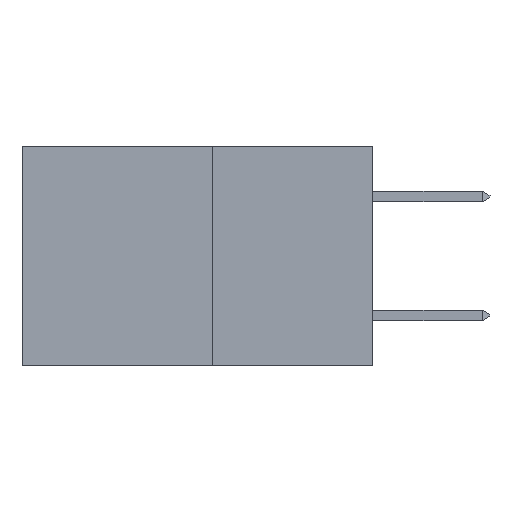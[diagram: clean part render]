
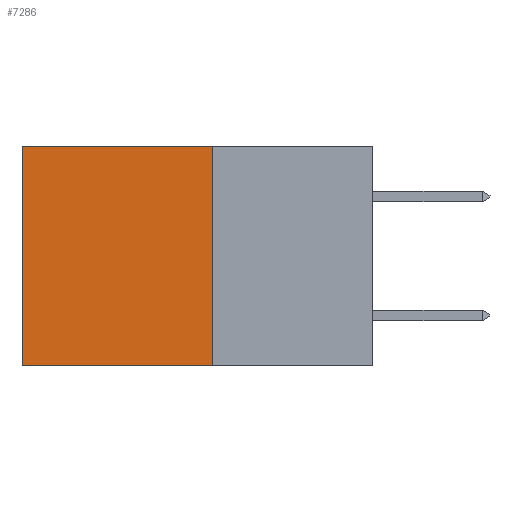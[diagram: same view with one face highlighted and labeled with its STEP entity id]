
A CAD part, left-side view. The second image highlights one B-rep face of the part: STEP entity #7286.
In plain terms, the highlighted planar face has unit normal (-1, 0, 0).
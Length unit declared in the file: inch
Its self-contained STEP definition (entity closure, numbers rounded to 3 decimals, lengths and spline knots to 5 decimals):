
#212 = LINE ( 'NONE', #3777, #11324 ) ;
#444 = CARTESIAN_POINT ( 'NONE',  ( 0.277, 0.27, -0.37 ) ) ;
#1114 = ORIENTED_EDGE ( 'NONE', *, *, #1220, .F. ) ;
#1220 = EDGE_CURVE ( 'NONE', #12785, #11777, #10015, .T. ) ;
#1423 = VERTEX_POINT ( 'NONE', #11241 ) ;
#1479 = AXIS2_PLACEMENT_3D ( 'NONE', #10381, #12316, #6412 ) ;
#1875 = FACE_OUTER_BOUND ( 'NONE', #11082, .T. ) ;
#2586 = LINE ( 'NONE', #10477, #10110 ) ;
#2786 = VERTEX_POINT ( 'NONE', #11202 ) ;
#3022 = EDGE_CURVE ( 'NONE', #2786, #12785, #11637, .T. ) ;
#3646 = CARTESIAN_POINT ( 'NONE',  ( 0.277, 0.27, -0.37 ) ) ;
#3752 = EDGE_CURVE ( 'NONE', #2786, #1423, #212, .T. ) ;
#3777 = CARTESIAN_POINT ( 'NONE',  ( 0.277, 0.27, 0. ) ) ;
#4813 = DIRECTION ( 'NONE',  ( 0., 1., 0. ) ) ;
#5529 = DIRECTION ( 'NONE',  ( 0., 0., -1. ) ) ;
#5591 = CARTESIAN_POINT ( 'NONE',  ( 0.277, 0.59, -0.37 ) ) ;
#6346 = VECTOR ( 'NONE', #10533, 39.37008 ) ;
#6412 = DIRECTION ( 'NONE',  ( 0., 0., -1. ) ) ;
#6817 = ORIENTED_EDGE ( 'NONE', *, *, #3022, .F. ) ;
#7286 = ADVANCED_FACE ( 'NONE', ( #1875 ), #9343, .F. ) ;
#9343 = PLANE ( 'NONE',  #1479 ) ;
#9415 = ORIENTED_EDGE ( 'NONE', *, *, #3752, .T. ) ;
#9535 = CARTESIAN_POINT ( 'NONE',  ( 0.277, 0.27, -0.37 ) ) ;
#9672 = VECTOR ( 'NONE', #12579, 39.37008 ) ;
#10015 = LINE ( 'NONE', #444, #9672 ) ;
#10110 = VECTOR ( 'NONE', #5529, 39.37008 ) ;
#10329 = EDGE_CURVE ( 'NONE', #1423, #11777, #2586, .T. ) ;
#10381 = CARTESIAN_POINT ( 'NONE',  ( 0.277, 0.27, -0.37 ) ) ;
#10477 = CARTESIAN_POINT ( 'NONE',  ( 0.277, 0.59, -0.37 ) ) ;
#10533 = DIRECTION ( 'NONE',  ( 0., 0., -1. ) ) ;
#11082 = EDGE_LOOP ( 'NONE', ( #11769, #1114, #6817, #9415 ) ) ;
#11202 = CARTESIAN_POINT ( 'NONE',  ( 0.277, 0.27, 0. ) ) ;
#11241 = CARTESIAN_POINT ( 'NONE',  ( 0.277, 0.59, 0. ) ) ;
#11324 = VECTOR ( 'NONE', #4813, 39.37008 ) ;
#11637 = LINE ( 'NONE', #9535, #6346 ) ;
#11769 = ORIENTED_EDGE ( 'NONE', *, *, #10329, .T. ) ;
#11777 = VERTEX_POINT ( 'NONE', #5591 ) ;
#12316 = DIRECTION ( 'NONE',  ( 1., 0., 0. ) ) ;
#12579 = DIRECTION ( 'NONE',  ( 0., 1., 0. ) ) ;
#12785 = VERTEX_POINT ( 'NONE', #3646 ) ;
